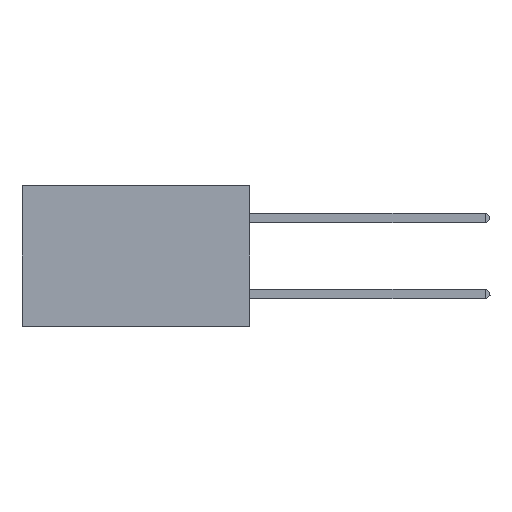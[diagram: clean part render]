
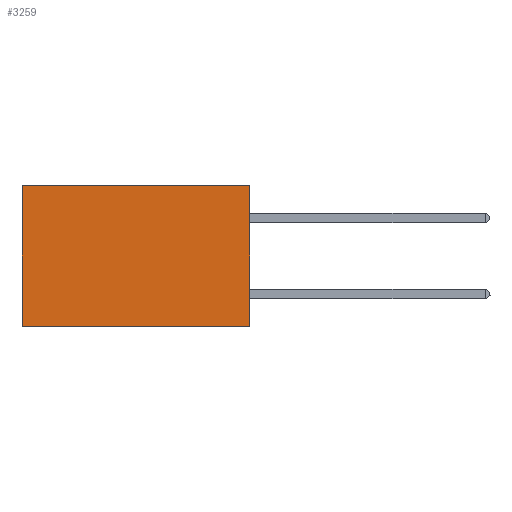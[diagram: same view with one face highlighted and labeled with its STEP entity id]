
A CAD part, left-side view. The second image highlights one B-rep face of the part: STEP entity #3259.
In plain terms, the highlighted planar face has unit normal (-1, 0, 0).
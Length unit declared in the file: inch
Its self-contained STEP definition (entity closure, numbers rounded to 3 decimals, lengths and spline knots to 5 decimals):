
#257 = CARTESIAN_POINT ( 'NONE',  ( 0.2875, 0.6, 0. ) ) ;
#1585 = EDGE_CURVE ( 'NONE', #5726, #11934, #8453, .T. ) ;
#2038 = EDGE_CURVE ( 'NONE', #7790, #10637, #7532, .T. ) ;
#2324 = DIRECTION ( 'NONE',  ( 0., 1., 0. ) ) ;
#2676 = ORIENTED_EDGE ( 'NONE', *, *, #13066, .T. ) ;
#3259 = ADVANCED_FACE ( 'NONE', ( #6406 ), #14799, .F. ) ;
#3493 = EDGE_CURVE ( 'NONE', #5726, #7790, #8781, .T. ) ;
#3679 = DIRECTION ( 'NONE',  ( 0., 0., -1. ) ) ;
#4111 = ORIENTED_EDGE ( 'NONE', *, *, #2038, .F. ) ;
#5726 = VERTEX_POINT ( 'NONE', #13998 ) ;
#6406 = FACE_OUTER_BOUND ( 'NONE', #8047, .T. ) ;
#6825 = ORIENTED_EDGE ( 'NONE', *, *, #1585, .T. ) ;
#7532 = LINE ( 'NONE', #13926, #11208 ) ;
#7790 = VERTEX_POINT ( 'NONE', #11947 ) ;
#8047 = EDGE_LOOP ( 'NONE', ( #2676, #4111, #13498, #6825 ) ) ;
#8453 = LINE ( 'NONE', #13654, #9400 ) ;
#8781 = LINE ( 'NONE', #11929, #11840 ) ;
#9334 = CARTESIAN_POINT ( 'NONE',  ( 0.2875, 0.6, -0.37 ) ) ;
#9400 = VECTOR ( 'NONE', #2324, 39.37008 ) ;
#10210 = CARTESIAN_POINT ( 'NONE',  ( 0.2875, 0.6, 0. ) ) ;
#10331 = DIRECTION ( 'NONE',  ( 0., 0., -1. ) ) ;
#10637 = VERTEX_POINT ( 'NONE', #9334 ) ;
#11055 = CARTESIAN_POINT ( 'NONE',  ( 0.2875, 0., 0. ) ) ;
#11104 = LINE ( 'NONE', #257, #11984 ) ;
#11208 = VECTOR ( 'NONE', #15111, 39.37008 ) ;
#11491 = AXIS2_PLACEMENT_3D ( 'NONE', #11055, #12543, #10331 ) ;
#11840 = VECTOR ( 'NONE', #3679, 39.37008 ) ;
#11929 = CARTESIAN_POINT ( 'NONE',  ( 0.2875, 0., 0. ) ) ;
#11934 = VERTEX_POINT ( 'NONE', #10210 ) ;
#11947 = CARTESIAN_POINT ( 'NONE',  ( 0.2875, 0., -0.37 ) ) ;
#11984 = VECTOR ( 'NONE', #12917, 39.37008 ) ;
#12543 = DIRECTION ( 'NONE',  ( 1., 0., 0. ) ) ;
#12917 = DIRECTION ( 'NONE',  ( 0., 0., -1. ) ) ;
#13066 = EDGE_CURVE ( 'NONE', #11934, #10637, #11104, .T. ) ;
#13498 = ORIENTED_EDGE ( 'NONE', *, *, #3493, .F. ) ;
#13654 = CARTESIAN_POINT ( 'NONE',  ( 0.2875, 0., 0. ) ) ;
#13926 = CARTESIAN_POINT ( 'NONE',  ( 0.2875, 0., -0.37 ) ) ;
#13998 = CARTESIAN_POINT ( 'NONE',  ( 0.2875, 0., 0. ) ) ;
#14799 = PLANE ( 'NONE',  #11491 ) ;
#15111 = DIRECTION ( 'NONE',  ( 0., 1., 0. ) ) ;
